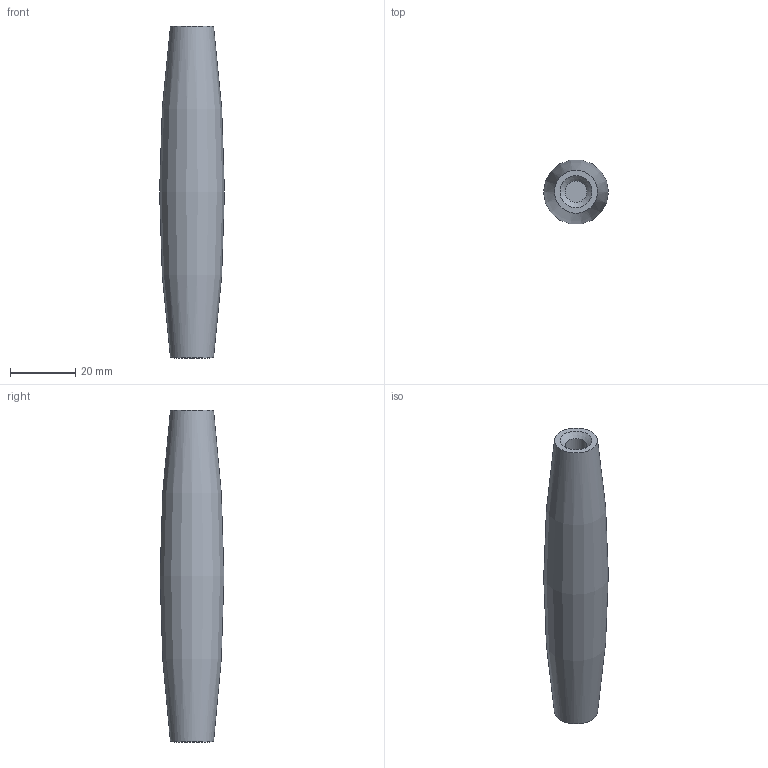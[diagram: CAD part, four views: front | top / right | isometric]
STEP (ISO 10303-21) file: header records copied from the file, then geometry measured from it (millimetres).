
FILE_DESCRIPTION(('FreeCAD Model'),'2;1');
FILE_NAME( 'DAVID-hand.step', '2018-08-24T11:17:54',('Author'),(''), 'Open CASCADE STEP processor 6.8','FreeCAD','Unknown');
FILE_SCHEMA(('AUTOMOTIVE_DESIGN_CC2 { 1 2 10303 214 -1 1 5 4 }'));
Length unit declared in the file: millimetre
Products named in the file (1): Chamfer
Bounding box: 19.84 x 19.54 x 101.6 mm (x, y, z)
Volume: 24534.9 mm3; surface area: 6200.3 mm2
Topology: 1 solids, 1 shells, 9 faces, 13 edges, 8 vertices
Faces by surface type: plane 4, cylinder 2, cone 2, revolution 1
Full cylindrical faces by diameter (mm): 6.604 x2
Entity records: 390 total; most frequent: DIRECTION 65, CARTESIAN_POINT 62, ORIENTED_EDGE 26, PCURVE 26, DEFINITIONAL_REPRESENTATION 26, LINE 20, VECTOR 20, AXIS2_PLACEMENT_3D 19
